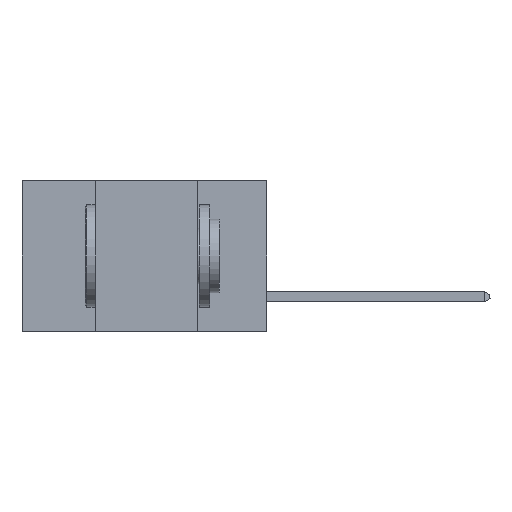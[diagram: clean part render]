
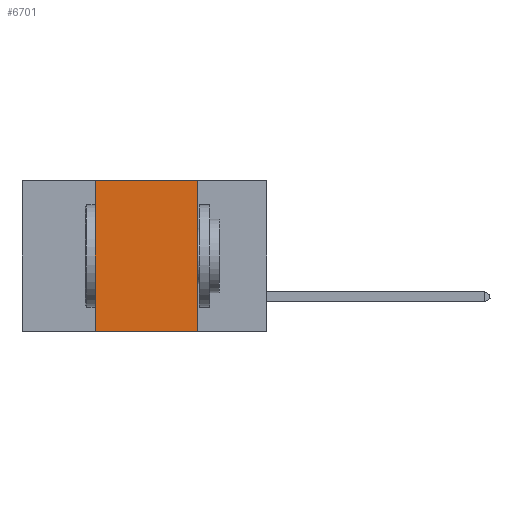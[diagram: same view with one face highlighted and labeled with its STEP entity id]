
A CAD part, left-side view. The second image highlights one B-rep face of the part: STEP entity #6701.
In plain terms, the highlighted planar face has unit normal (-1, 0, 0).
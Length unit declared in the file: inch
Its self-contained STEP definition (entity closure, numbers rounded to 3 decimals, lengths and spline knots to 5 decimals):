
#425 = VERTEX_POINT ( 'NONE', #7723 ) ;
#841 = VERTEX_POINT ( 'NONE', #2680 ) ;
#1620 = CARTESIAN_POINT ( 'NONE',  ( 0., 0.6, 0. ) ) ;
#2224 = CARTESIAN_POINT ( 'NONE',  ( 0., 0.17, 0. ) ) ;
#2505 = DIRECTION ( 'NONE',  ( 0., 0., 1. ) ) ;
#2619 = DIRECTION ( 'NONE',  ( 0., -1., 0. ) ) ;
#2680 = CARTESIAN_POINT ( 'NONE',  ( 0., 0.17, -0.37 ) ) ;
#2739 = VECTOR ( 'NONE', #8643, 39.37008 ) ;
#2830 = FACE_OUTER_BOUND ( 'NONE', #7710, .T. ) ;
#3197 = LINE ( 'NONE', #9639, #3444 ) ;
#3444 = VECTOR ( 'NONE', #2619, 39.37008 ) ;
#3585 = EDGE_CURVE ( 'NONE', #9688, #841, #7543, .T. ) ;
#4467 = VECTOR ( 'NONE', #5432, 39.37008 ) ;
#4607 = VERTEX_POINT ( 'NONE', #5628 ) ;
#4690 = PLANE ( 'NONE',  #7100 ) ;
#5432 = DIRECTION ( 'NONE',  ( 0., 0., -1. ) ) ;
#5532 = EDGE_CURVE ( 'NONE', #425, #841, #7673, .T. ) ;
#5536 = DIRECTION ( 'NONE',  ( 0., 0., -1. ) ) ;
#5628 = CARTESIAN_POINT ( 'NONE',  ( 0., 0.42, 0. ) ) ;
#5764 = LINE ( 'NONE', #7205, #7365 ) ;
#6701 = ADVANCED_FACE ( 'NONE', ( #2830 ), #4690, .F. ) ;
#7100 = AXIS2_PLACEMENT_3D ( 'NONE', #1620, #10156, #5536 ) ;
#7205 = CARTESIAN_POINT ( 'NONE',  ( 0., 0.42, 0. ) ) ;
#7365 = VECTOR ( 'NONE', #2505, 39.37008 ) ;
#7543 = LINE ( 'NONE', #2224, #4467 ) ;
#7673 = LINE ( 'NONE', #7929, #2739 ) ;
#7710 = EDGE_LOOP ( 'NONE', ( #8262, #8140, #10120, #8844 ) ) ;
#7723 = CARTESIAN_POINT ( 'NONE',  ( 0., 0.42, -0.37 ) ) ;
#7775 = EDGE_CURVE ( 'NONE', #425, #4607, #5764, .T. ) ;
#7786 = CARTESIAN_POINT ( 'NONE',  ( 0., 0.17, 0. ) ) ;
#7929 = CARTESIAN_POINT ( 'NONE',  ( 0., 0.6, -0.37 ) ) ;
#8140 = ORIENTED_EDGE ( 'NONE', *, *, #9327, .F. ) ;
#8262 = ORIENTED_EDGE ( 'NONE', *, *, #3585, .F. ) ;
#8643 = DIRECTION ( 'NONE',  ( 0., -1., 0. ) ) ;
#8844 = ORIENTED_EDGE ( 'NONE', *, *, #5532, .T. ) ;
#9327 = EDGE_CURVE ( 'NONE', #4607, #9688, #3197, .T. ) ;
#9639 = CARTESIAN_POINT ( 'NONE',  ( 0., 0.6, 0. ) ) ;
#9688 = VERTEX_POINT ( 'NONE', #7786 ) ;
#10120 = ORIENTED_EDGE ( 'NONE', *, *, #7775, .F. ) ;
#10156 = DIRECTION ( 'NONE',  ( 1., 0., 0. ) ) ;
